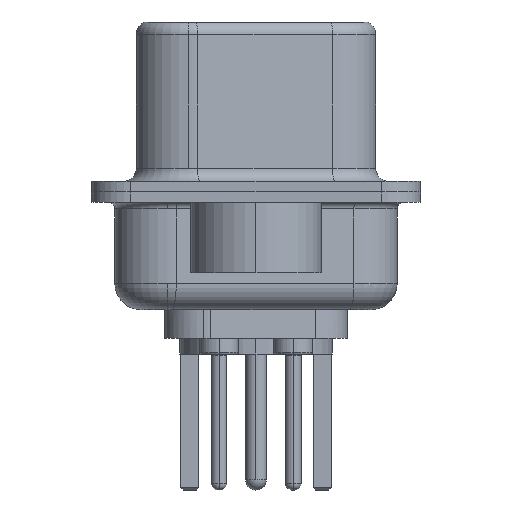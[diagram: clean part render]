
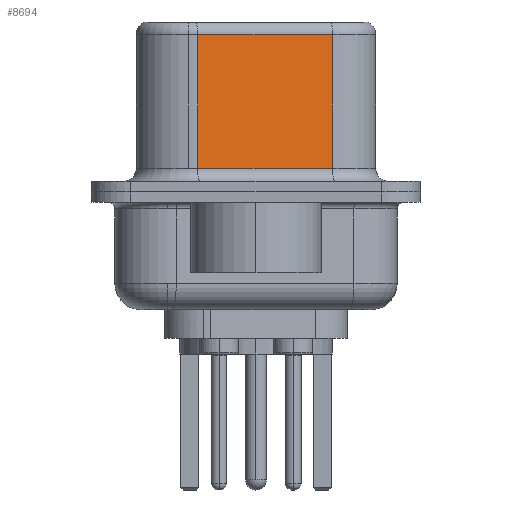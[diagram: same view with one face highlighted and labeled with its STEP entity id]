
A CAD part, left-side view. The second image highlights one B-rep face of the part: STEP entity #8694.
In plain terms, the highlighted planar face has unit normal (-0.985, -0.174, 0).
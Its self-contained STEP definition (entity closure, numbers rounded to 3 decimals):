
#272 = CARTESIAN_POINT ( 'NONE',  ( 3.655, 2.233, 6.52 ) ) ;
#497 = ORIENTED_EDGE ( 'NONE', *, *, #1438, .T. ) ;
#1438 = EDGE_CURVE ( 'NONE', #9365, #11138, #14784, .T. ) ;
#1709 = DIRECTION ( 'NONE',  ( 0., 0., -1. ) ) ;
#1746 = ORIENTED_EDGE ( 'NONE', *, *, #2219, .F. ) ;
#1976 = LINE ( 'NONE', #2357, #16790 ) ;
#2082 = EDGE_LOOP ( 'NONE', ( #1746, #6798, #497, #8140 ) ) ;
#2219 = EDGE_CURVE ( 'NONE', #10754, #12649, #6619, .T. ) ;
#2357 = CARTESIAN_POINT ( 'NONE',  ( 4.565, -2.927, 6.02 ) ) ;
#3990 = CARTESIAN_POINT ( 'NONE',  ( 4.565, -2.927, 0.9 ) ) ;
#6619 = LINE ( 'NONE', #15011, #18200 ) ;
#6798 = ORIENTED_EDGE ( 'NONE', *, *, #8406, .T. ) ;
#6916 = DIRECTION ( 'NONE',  ( 0., 0., -1. ) ) ;
#7144 = CARTESIAN_POINT ( 'NONE',  ( 3.655, 2.233, 0.9 ) ) ;
#7560 = CARTESIAN_POINT ( 'NONE',  ( 4.565, -2.927, 6.02 ) ) ;
#8140 = ORIENTED_EDGE ( 'NONE', *, *, #10603, .T. ) ;
#8406 = EDGE_CURVE ( 'NONE', #10754, #9365, #1976, .T. ) ;
#8694 = ADVANCED_FACE ( 'NONE', ( #18361 ), #13823, .F. ) ;
#9365 = VERTEX_POINT ( 'NONE', #18251 ) ;
#10481 = DIRECTION ( 'NONE',  ( -0.174, 0.985, 0. ) ) ;
#10603 = EDGE_CURVE ( 'NONE', #11138, #12649, #11098, .T. ) ;
#10614 = DIRECTION ( 'NONE',  ( -0.174, 0.985, 0. ) ) ;
#10754 = VERTEX_POINT ( 'NONE', #7560 ) ;
#10762 = VECTOR ( 'NONE', #6916, 1000. ) ;
#11098 = LINE ( 'NONE', #14769, #14644 ) ;
#11138 = VERTEX_POINT ( 'NONE', #7144 ) ;
#12649 = VERTEX_POINT ( 'NONE', #3990 ) ;
#12938 = AXIS2_PLACEMENT_3D ( 'NONE', #17703, #13777, #10614 ) ;
#13777 = DIRECTION ( 'NONE',  ( 0.985, 0.174, 0. ) ) ;
#13823 = PLANE ( 'NONE',  #12938 ) ;
#14644 = VECTOR ( 'NONE', #16022, 1000. ) ;
#14769 = CARTESIAN_POINT ( 'NONE',  ( 4.565, -2.927, 0.9 ) ) ;
#14784 = LINE ( 'NONE', #272, #10762 ) ;
#15011 = CARTESIAN_POINT ( 'NONE',  ( 4.565, -2.927, 6.52 ) ) ;
#16022 = DIRECTION ( 'NONE',  ( 0.174, -0.985, 0. ) ) ;
#16790 = VECTOR ( 'NONE', #10481, 1000. ) ;
#17703 = CARTESIAN_POINT ( 'NONE',  ( 4.565, -2.927, 6.52 ) ) ;
#18200 = VECTOR ( 'NONE', #1709, 1000. ) ;
#18251 = CARTESIAN_POINT ( 'NONE',  ( 3.655, 2.233, 6.02 ) ) ;
#18361 = FACE_OUTER_BOUND ( 'NONE', #2082, .T. ) ;
